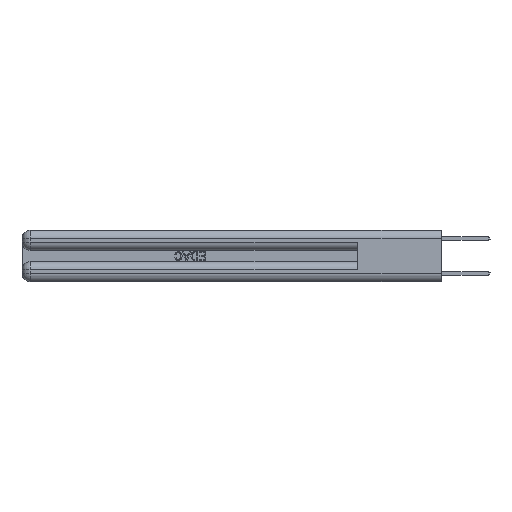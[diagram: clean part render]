
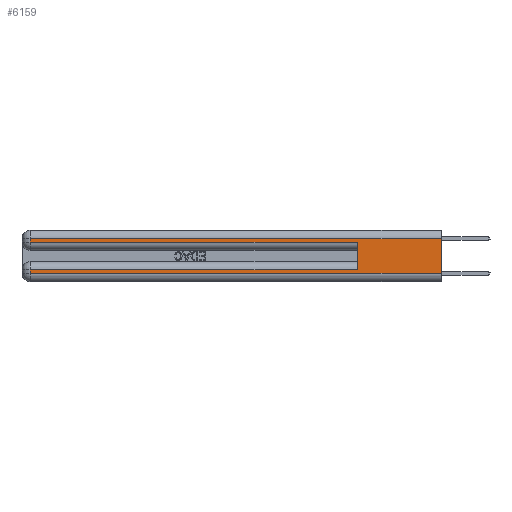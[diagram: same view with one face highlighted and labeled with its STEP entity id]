
A CAD part, left-side view. The second image highlights one B-rep face of the part: STEP entity #6159.
In plain terms, the highlighted planar face has unit normal (-1, 0, 0).
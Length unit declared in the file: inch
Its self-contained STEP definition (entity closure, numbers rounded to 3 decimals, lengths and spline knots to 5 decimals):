
#490 = CARTESIAN_POINT ( 'NONE',  ( 0., 0., 0.06 ) ) ;
#614 = ORIENTED_EDGE ( 'NONE', *, *, #22464, .T. ) ;
#1136 = EDGE_CURVE ( 'NONE', #22821, #30769, #7209, .T. ) ;
#1383 = EDGE_CURVE ( 'NONE', #21060, #35211, #35215, .T. ) ;
#2088 = FACE_OUTER_BOUND ( 'NONE', #5508, .T. ) ;
#2434 = CARTESIAN_POINT ( 'NONE',  ( 0., 0., 0.085 ) ) ;
#2549 = DIRECTION ( 'NONE',  ( 0., 0., 1. ) ) ;
#3187 = CARTESIAN_POINT ( 'NONE',  ( 0., 0., 0.31 ) ) ;
#3819 = LINE ( 'NONE', #17251, #8258 ) ;
#4068 = VERTEX_POINT ( 'NONE', #33648 ) ;
#4554 = CARTESIAN_POINT ( 'NONE',  ( 0., 0., 0.285 ) ) ;
#5479 = ORIENTED_EDGE ( 'NONE', *, *, #28806, .T. ) ;
#5508 = EDGE_LOOP ( 'NONE', ( #18856, #18348, #12706, #26704, #15251, #614, #5479, #8893 ) ) ;
#6159 = ADVANCED_FACE ( 'NONE', ( #2088 ), #27038, .F. ) ;
#6381 = VECTOR ( 'NONE', #15589, 39.37008 ) ;
#7209 = LINE ( 'NONE', #23928, #11681 ) ;
#8258 = VECTOR ( 'NONE', #11698, 39.37008 ) ;
#8295 = VECTOR ( 'NONE', #27360, 39.37008 ) ;
#8893 = ORIENTED_EDGE ( 'NONE', *, *, #18944, .T. ) ;
#8991 = CARTESIAN_POINT ( 'NONE',  ( 0., 2.94, 0.085 ) ) ;
#10690 = CARTESIAN_POINT ( 'NONE',  ( 0., 2.94, 0.37 ) ) ;
#11029 = VECTOR ( 'NONE', #24203, 39.37008 ) ;
#11681 = VECTOR ( 'NONE', #15597, 39.37008 ) ;
#11698 = DIRECTION ( 'NONE',  ( 0., 1., 0. ) ) ;
#12190 = VECTOR ( 'NONE', #28999, 39.37008 ) ;
#12706 = ORIENTED_EDGE ( 'NONE', *, *, #16983, .T. ) ;
#15177 = CARTESIAN_POINT ( 'NONE',  ( 0., 2.94, 0.285 ) ) ;
#15251 = ORIENTED_EDGE ( 'NONE', *, *, #1383, .F. ) ;
#15589 = DIRECTION ( 'NONE',  ( 0., -1., 0. ) ) ;
#15597 = DIRECTION ( 'NONE',  ( 0., 0., -1. ) ) ;
#15941 = DIRECTION ( 'NONE',  ( 0., 0., -1. ) ) ;
#16188 = CARTESIAN_POINT ( 'NONE',  ( 0., 0., 0.37 ) ) ;
#16780 = CARTESIAN_POINT ( 'NONE',  ( 0., 0.6, 0.285 ) ) ;
#16869 = VERTEX_POINT ( 'NONE', #15177 ) ;
#16941 = LINE ( 'NONE', #10690, #27377 ) ;
#16983 = EDGE_CURVE ( 'NONE', #18230, #16869, #31163, .T. ) ;
#17251 = CARTESIAN_POINT ( 'NONE',  ( 0., 0., 0.31 ) ) ;
#18230 = VERTEX_POINT ( 'NONE', #18745 ) ;
#18348 = ORIENTED_EDGE ( 'NONE', *, *, #23028, .T. ) ;
#18745 = CARTESIAN_POINT ( 'NONE',  ( 0., 2.94, 0.31 ) ) ;
#18856 = ORIENTED_EDGE ( 'NONE', *, *, #1136, .F. ) ;
#18944 = EDGE_CURVE ( 'NONE', #4068, #30769, #25806, .T. ) ;
#19129 = DIRECTION ( 'NONE',  ( 0., 0., -1. ) ) ;
#20167 = CARTESIAN_POINT ( 'NONE',  ( 0., 0., 0.06 ) ) ;
#20437 = VERTEX_POINT ( 'NONE', #8991 ) ;
#21060 = VERTEX_POINT ( 'NONE', #21686 ) ;
#21686 = CARTESIAN_POINT ( 'NONE',  ( 0., 0.6, 0.085 ) ) ;
#22464 = EDGE_CURVE ( 'NONE', #21060, #20437, #25053, .T. ) ;
#22821 = VERTEX_POINT ( 'NONE', #3187 ) ;
#23028 = EDGE_CURVE ( 'NONE', #22821, #18230, #3819, .T. ) ;
#23928 = CARTESIAN_POINT ( 'NONE',  ( 0., 0., 0.37 ) ) ;
#24203 = DIRECTION ( 'NONE',  ( 0., 0., -1. ) ) ;
#24437 = CARTESIAN_POINT ( 'NONE',  ( 0., 2.94, 0.37 ) ) ;
#24581 = CARTESIAN_POINT ( 'NONE',  ( 0., 0.6, 0.145 ) ) ;
#25053 = LINE ( 'NONE', #2434, #8295 ) ;
#25806 = LINE ( 'NONE', #20167, #12190 ) ;
#26704 = ORIENTED_EDGE ( 'NONE', *, *, #33407, .T. ) ;
#27038 = PLANE ( 'NONE',  #29647 ) ;
#27360 = DIRECTION ( 'NONE',  ( 0., 1., 0. ) ) ;
#27377 = VECTOR ( 'NONE', #19129, 39.37008 ) ;
#27510 = DIRECTION ( 'NONE',  ( 1., 0., 0. ) ) ;
#28806 = EDGE_CURVE ( 'NONE', #20437, #4068, #16941, .T. ) ;
#28999 = DIRECTION ( 'NONE',  ( 0., -1., 0. ) ) ;
#29647 = AXIS2_PLACEMENT_3D ( 'NONE', #16188, #27510, #15941 ) ;
#30769 = VERTEX_POINT ( 'NONE', #490 ) ;
#31163 = LINE ( 'NONE', #24437, #11029 ) ;
#33114 = VECTOR ( 'NONE', #2549, 39.37008 ) ;
#33407 = EDGE_CURVE ( 'NONE', #16869, #35211, #36242, .T. ) ;
#33648 = CARTESIAN_POINT ( 'NONE',  ( 0., 2.94, 0.06 ) ) ;
#35211 = VERTEX_POINT ( 'NONE', #16780 ) ;
#35215 = LINE ( 'NONE', #24581, #33114 ) ;
#36242 = LINE ( 'NONE', #4554, #6381 ) ;
